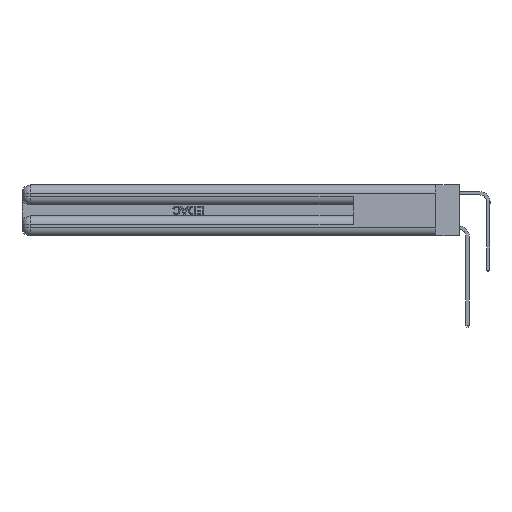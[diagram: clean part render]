
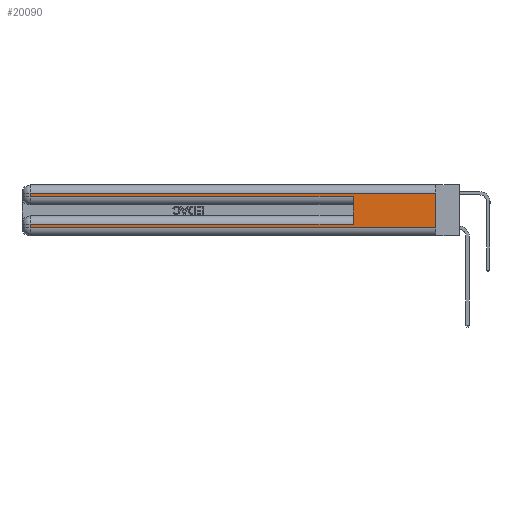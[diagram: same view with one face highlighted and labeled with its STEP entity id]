
A CAD part, left-side view. The second image highlights one B-rep face of the part: STEP entity #20090.
In plain terms, the highlighted planar face has unit normal (-1, 0, 0).
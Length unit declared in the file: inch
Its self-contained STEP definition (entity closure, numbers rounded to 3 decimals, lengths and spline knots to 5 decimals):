
#578 = CARTESIAN_POINT ( 'NONE',  ( 0., 2.94, 0.06 ) ) ;
#643 = DIRECTION ( 'NONE',  ( 0., -1., 0. ) ) ;
#921 = CARTESIAN_POINT ( 'NONE',  ( 0., 0., 0.085 ) ) ;
#1019 = DIRECTION ( 'NONE',  ( 1., 0., 0. ) ) ;
#3257 = LINE ( 'NONE', #921, #20950 ) ;
#3725 = PLANE ( 'NONE',  #14968 ) ;
#4770 = VERTEX_POINT ( 'NONE', #21990 ) ;
#4778 = ORIENTED_EDGE ( 'NONE', *, *, #24099, .F. ) ;
#4950 = CARTESIAN_POINT ( 'NONE',  ( 0., 0.6, 0.145 ) ) ;
#5519 = CARTESIAN_POINT ( 'NONE',  ( 0., 2.94, 0.31 ) ) ;
#5715 = CARTESIAN_POINT ( 'NONE',  ( 0., 0., 0.06 ) ) ;
#5752 = ORIENTED_EDGE ( 'NONE', *, *, #8839, .T. ) ;
#6135 = ORIENTED_EDGE ( 'NONE', *, *, #28163, .T. ) ;
#6766 = VECTOR ( 'NONE', #643, 39.37008 ) ;
#6815 = CARTESIAN_POINT ( 'NONE',  ( 0., 0., 0.37 ) ) ;
#7073 = CARTESIAN_POINT ( 'NONE',  ( 0., 0., 0.31 ) ) ;
#7172 = DIRECTION ( 'NONE',  ( 0., 0., -1. ) ) ;
#7192 = CARTESIAN_POINT ( 'NONE',  ( 0., 0., 0.285 ) ) ;
#7257 = DIRECTION ( 'NONE',  ( 0., 1., 0. ) ) ;
#7787 = VECTOR ( 'NONE', #25969, 39.37008 ) ;
#8124 = VERTEX_POINT ( 'NONE', #5519 ) ;
#8449 = VERTEX_POINT ( 'NONE', #36687 ) ;
#8750 = DIRECTION ( 'NONE',  ( 0., 0., -1. ) ) ;
#8839 = EDGE_CURVE ( 'NONE', #8124, #17786, #27986, .T. ) ;
#9240 = VERTEX_POINT ( 'NONE', #578 ) ;
#9994 = LINE ( 'NONE', #30235, #25127 ) ;
#10106 = FACE_OUTER_BOUND ( 'NONE', #11229, .T. ) ;
#11126 = EDGE_CURVE ( 'NONE', #9240, #12080, #9994, .T. ) ;
#11132 = VECTOR ( 'NONE', #7257, 39.37008 ) ;
#11229 = EDGE_LOOP ( 'NONE', ( #19345, #32116, #5752, #31275, #4778, #6135, #22920, #17592 ) ) ;
#12080 = VERTEX_POINT ( 'NONE', #5715 ) ;
#14871 = EDGE_CURVE ( 'NONE', #17786, #8449, #15884, .T. ) ;
#14968 = AXIS2_PLACEMENT_3D ( 'NONE', #6815, #1019, #18400 ) ;
#15105 = VERTEX_POINT ( 'NONE', #19159 ) ;
#15241 = EDGE_CURVE ( 'NONE', #16581, #9240, #17999, .T. ) ;
#15688 = EDGE_CURVE ( 'NONE', #4770, #8124, #33480, .T. ) ;
#15884 = LINE ( 'NONE', #7192, #6766 ) ;
#16581 = VERTEX_POINT ( 'NONE', #29087 ) ;
#17444 = CARTESIAN_POINT ( 'NONE',  ( 0., 0., 0.37 ) ) ;
#17470 = EDGE_CURVE ( 'NONE', #4770, #12080, #32265, .T. ) ;
#17592 = ORIENTED_EDGE ( 'NONE', *, *, #11126, .T. ) ;
#17786 = VERTEX_POINT ( 'NONE', #28526 ) ;
#17999 = LINE ( 'NONE', #32047, #28950 ) ;
#18306 = DIRECTION ( 'NONE',  ( 0., 1., 0. ) ) ;
#18400 = DIRECTION ( 'NONE',  ( 0., 0., -1. ) ) ;
#19159 = CARTESIAN_POINT ( 'NONE',  ( 0., 0.6, 0.085 ) ) ;
#19345 = ORIENTED_EDGE ( 'NONE', *, *, #17470, .F. ) ;
#20090 = ADVANCED_FACE ( 'NONE', ( #10106 ), #3725, .F. ) ;
#20950 = VECTOR ( 'NONE', #18306, 39.37008 ) ;
#21567 = DIRECTION ( 'NONE',  ( 0., -1., 0. ) ) ;
#21990 = CARTESIAN_POINT ( 'NONE',  ( 0., 0., 0.31 ) ) ;
#22700 = LINE ( 'NONE', #4950, #7787 ) ;
#22920 = ORIENTED_EDGE ( 'NONE', *, *, #15241, .T. ) ;
#24099 = EDGE_CURVE ( 'NONE', #15105, #8449, #22700, .T. ) ;
#25127 = VECTOR ( 'NONE', #21567, 39.37008 ) ;
#25969 = DIRECTION ( 'NONE',  ( 0., 0., 1. ) ) ;
#27986 = LINE ( 'NONE', #36458, #32506 ) ;
#28163 = EDGE_CURVE ( 'NONE', #15105, #16581, #3257, .T. ) ;
#28526 = CARTESIAN_POINT ( 'NONE',  ( 0., 2.94, 0.285 ) ) ;
#28950 = VECTOR ( 'NONE', #29156, 39.37008 ) ;
#29087 = CARTESIAN_POINT ( 'NONE',  ( 0., 2.94, 0.085 ) ) ;
#29156 = DIRECTION ( 'NONE',  ( 0., 0., -1. ) ) ;
#30235 = CARTESIAN_POINT ( 'NONE',  ( 0., 0., 0.06 ) ) ;
#31275 = ORIENTED_EDGE ( 'NONE', *, *, #14871, .T. ) ;
#32047 = CARTESIAN_POINT ( 'NONE',  ( 0., 2.94, 0.37 ) ) ;
#32116 = ORIENTED_EDGE ( 'NONE', *, *, #15688, .T. ) ;
#32265 = LINE ( 'NONE', #17444, #35848 ) ;
#32506 = VECTOR ( 'NONE', #7172, 39.37008 ) ;
#33480 = LINE ( 'NONE', #7073, #11132 ) ;
#35848 = VECTOR ( 'NONE', #8750, 39.37008 ) ;
#36458 = CARTESIAN_POINT ( 'NONE',  ( 0., 2.94, 0.37 ) ) ;
#36687 = CARTESIAN_POINT ( 'NONE',  ( 0., 0.6, 0.285 ) ) ;
